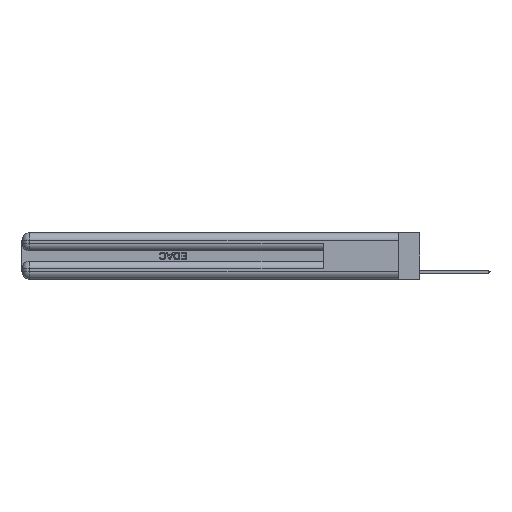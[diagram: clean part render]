
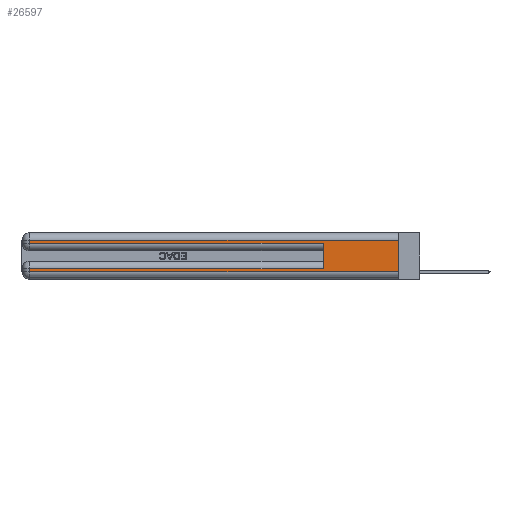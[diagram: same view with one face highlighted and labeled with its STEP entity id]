
A CAD part, left-side view. The second image highlights one B-rep face of the part: STEP entity #26597.
In plain terms, the highlighted planar face has unit normal (-1, 0, 0).
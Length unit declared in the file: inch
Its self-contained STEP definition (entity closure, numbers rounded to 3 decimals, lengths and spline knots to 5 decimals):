
#138 = EDGE_LOOP ( 'NONE', ( #27762, #25245, #12337, #341, #3847, #1339, #21164, #31731 ) ) ;
#341 = ORIENTED_EDGE ( 'NONE', *, *, #13558, .T. ) ;
#488 = CARTESIAN_POINT ( 'NONE',  ( 0., 2.94, 0.06 ) ) ;
#1339 = ORIENTED_EDGE ( 'NONE', *, *, #23888, .T. ) ;
#1365 = EDGE_CURVE ( 'NONE', #3404, #31573, #4242, .T. ) ;
#3103 = CARTESIAN_POINT ( 'NONE',  ( 0., 0., 0.31 ) ) ;
#3383 = VECTOR ( 'NONE', #21069, 39.37008 ) ;
#3404 = VERTEX_POINT ( 'NONE', #10659 ) ;
#3847 = ORIENTED_EDGE ( 'NONE', *, *, #21623, .F. ) ;
#4211 = DIRECTION ( 'NONE',  ( 0., 0., -1. ) ) ;
#4242 = LINE ( 'NONE', #19402, #27331 ) ;
#4461 = VERTEX_POINT ( 'NONE', #17935 ) ;
#4466 = AXIS2_PLACEMENT_3D ( 'NONE', #9267, #19366, #4211 ) ;
#4568 = DIRECTION ( 'NONE',  ( 0., 0., -1. ) ) ;
#4815 = VECTOR ( 'NONE', #28485, 39.37008 ) ;
#6011 = VERTEX_POINT ( 'NONE', #3103 ) ;
#6243 = EDGE_CURVE ( 'NONE', #6011, #28107, #21614, .T. ) ;
#6377 = CARTESIAN_POINT ( 'NONE',  ( 0., 0., 0.31 ) ) ;
#6442 = EDGE_CURVE ( 'NONE', #6011, #28944, #19345, .T. ) ;
#6731 = PLANE ( 'NONE',  #4466 ) ;
#7881 = VECTOR ( 'NONE', #28124, 39.37008 ) ;
#8192 = VECTOR ( 'NONE', #30921, 39.37008 ) ;
#8932 = FACE_OUTER_BOUND ( 'NONE', #138, .T. ) ;
#9235 = VERTEX_POINT ( 'NONE', #31019 ) ;
#9267 = CARTESIAN_POINT ( 'NONE',  ( 0., 0., 0.37 ) ) ;
#9324 = CARTESIAN_POINT ( 'NONE',  ( 0., 0., 0.37 ) ) ;
#10463 = CARTESIAN_POINT ( 'NONE',  ( 0., 2.94, 0.37 ) ) ;
#10659 = CARTESIAN_POINT ( 'NONE',  ( 0., 2.94, 0.085 ) ) ;
#11251 = VECTOR ( 'NONE', #19604, 39.37008 ) ;
#12185 = LINE ( 'NONE', #10463, #7881 ) ;
#12224 = EDGE_CURVE ( 'NONE', #28944, #4461, #12185, .T. ) ;
#12337 = ORIENTED_EDGE ( 'NONE', *, *, #12224, .T. ) ;
#12372 = LINE ( 'NONE', #22642, #8192 ) ;
#12523 = LINE ( 'NONE', #22794, #18489 ) ;
#13558 = EDGE_CURVE ( 'NONE', #4461, #22352, #12523, .T. ) ;
#15748 = EDGE_CURVE ( 'NONE', #31573, #28107, #12372, .T. ) ;
#16070 = CARTESIAN_POINT ( 'NONE',  ( 0., 2.94, 0.31 ) ) ;
#16181 = CARTESIAN_POINT ( 'NONE',  ( 0., 0., 0.085 ) ) ;
#17768 = DIRECTION ( 'NONE',  ( 0., -1., 0. ) ) ;
#17935 = CARTESIAN_POINT ( 'NONE',  ( 0., 2.94, 0.285 ) ) ;
#18489 = VECTOR ( 'NONE', #17768, 39.37008 ) ;
#19345 = LINE ( 'NONE', #6377, #4815 ) ;
#19366 = DIRECTION ( 'NONE',  ( 1., 0., 0. ) ) ;
#19402 = CARTESIAN_POINT ( 'NONE',  ( 0., 2.94, 0.37 ) ) ;
#19604 = DIRECTION ( 'NONE',  ( 0., 0., -1. ) ) ;
#21069 = DIRECTION ( 'NONE',  ( 0., 1., 0. ) ) ;
#21164 = ORIENTED_EDGE ( 'NONE', *, *, #1365, .T. ) ;
#21614 = LINE ( 'NONE', #9324, #11251 ) ;
#21623 = EDGE_CURVE ( 'NONE', #9235, #22352, #27536, .T. ) ;
#22352 = VERTEX_POINT ( 'NONE', #26138 ) ;
#22642 = CARTESIAN_POINT ( 'NONE',  ( 0., 0., 0.06 ) ) ;
#22794 = CARTESIAN_POINT ( 'NONE',  ( 0., 0., 0.285 ) ) ;
#23888 = EDGE_CURVE ( 'NONE', #9235, #3404, #23921, .T. ) ;
#23921 = LINE ( 'NONE', #16181, #3383 ) ;
#24184 = CARTESIAN_POINT ( 'NONE',  ( 0., 0.6, 0.145 ) ) ;
#24358 = DIRECTION ( 'NONE',  ( 0., 0., 1. ) ) ;
#25245 = ORIENTED_EDGE ( 'NONE', *, *, #6442, .T. ) ;
#25792 = CARTESIAN_POINT ( 'NONE',  ( 0., 0., 0.06 ) ) ;
#26138 = CARTESIAN_POINT ( 'NONE',  ( 0., 0.6, 0.285 ) ) ;
#26597 = ADVANCED_FACE ( 'NONE', ( #8932 ), #6731, .F. ) ;
#27331 = VECTOR ( 'NONE', #4568, 39.37008 ) ;
#27536 = LINE ( 'NONE', #24184, #33018 ) ;
#27762 = ORIENTED_EDGE ( 'NONE', *, *, #6243, .F. ) ;
#28107 = VERTEX_POINT ( 'NONE', #25792 ) ;
#28124 = DIRECTION ( 'NONE',  ( 0., 0., -1. ) ) ;
#28485 = DIRECTION ( 'NONE',  ( 0., 1., 0. ) ) ;
#28944 = VERTEX_POINT ( 'NONE', #16070 ) ;
#30921 = DIRECTION ( 'NONE',  ( 0., -1., 0. ) ) ;
#31019 = CARTESIAN_POINT ( 'NONE',  ( 0., 0.6, 0.085 ) ) ;
#31573 = VERTEX_POINT ( 'NONE', #488 ) ;
#31731 = ORIENTED_EDGE ( 'NONE', *, *, #15748, .T. ) ;
#33018 = VECTOR ( 'NONE', #24358, 39.37008 ) ;
